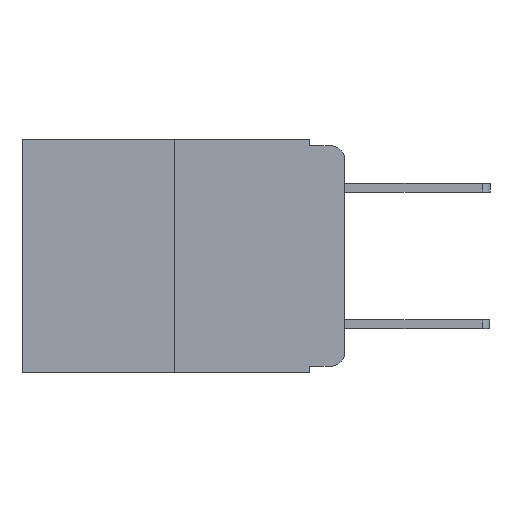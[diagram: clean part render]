
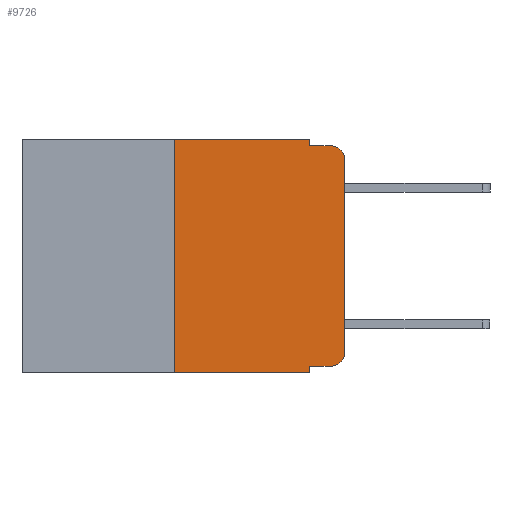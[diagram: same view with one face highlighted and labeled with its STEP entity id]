
A CAD part, left-side view. The second image highlights one B-rep face of the part: STEP entity #9726.
In plain terms, the highlighted planar face has unit normal (-1, 0, 0).
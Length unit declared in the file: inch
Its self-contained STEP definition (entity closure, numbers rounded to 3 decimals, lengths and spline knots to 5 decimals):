
#6 = EDGE_LOOP ( 'NONE', ( #5676, #11963, #8001, #12104, #3830, #6440, #8475, #7396, #10908, #8155 ) ) ;
#300 = FACE_OUTER_BOUND ( 'NONE', #6, .T. ) ;
#561 = VERTEX_POINT ( 'NONE', #10012 ) ;
#923 = CARTESIAN_POINT ( 'NONE',  ( 0., 0.473, -0.343 ) ) ;
#1143 = AXIS2_PLACEMENT_3D ( 'NONE', #9100, #2590, #10168 ) ;
#1240 = CARTESIAN_POINT ( 'NONE',  ( 0., 0.02, -0.03 ) ) ;
#1515 = DIRECTION ( 'NONE',  ( 0., -1., 0. ) ) ;
#1975 = LINE ( 'NONE', #8167, #10622 ) ;
#2472 = DIRECTION ( 'NONE',  ( 0., 0., -1. ) ) ;
#2590 = DIRECTION ( 'NONE',  ( -1., 0., 0. ) ) ;
#2690 = CARTESIAN_POINT ( 'NONE',  ( 0., 0.051, -0.333 ) ) ;
#2738 = VECTOR ( 'NONE', #5827, 39.37008 ) ;
#3162 = VERTEX_POINT ( 'NONE', #2690 ) ;
#3560 = CARTESIAN_POINT ( 'NONE',  ( 0., 0.02, -0.333 ) ) ;
#3591 = VERTEX_POINT ( 'NONE', #3560 ) ;
#3830 = ORIENTED_EDGE ( 'NONE', *, *, #11233, .F. ) ;
#3986 = PLANE ( 'NONE',  #9888 ) ;
#4048 = CIRCLE ( 'NONE', #1143, 0.02 ) ;
#4420 = LINE ( 'NONE', #9017, #10023 ) ;
#4457 = LINE ( 'NONE', #7107, #9730 ) ;
#4515 = DIRECTION ( 'NONE',  ( 0., -1., 0. ) ) ;
#4577 = EDGE_CURVE ( 'NONE', #561, #8342, #7917, .T. ) ;
#4603 = EDGE_CURVE ( 'NONE', #12995, #8988, #4457, .T. ) ;
#4677 = CARTESIAN_POINT ( 'NONE',  ( 0., 0.051, 0. ) ) ;
#4731 = CARTESIAN_POINT ( 'NONE',  ( 0., 0.051, 0. ) ) ;
#4931 = CARTESIAN_POINT ( 'NONE',  ( 0., 0.25, 0. ) ) ;
#5066 = VERTEX_POINT ( 'NONE', #13216 ) ;
#5166 = DIRECTION ( 'NONE',  ( 1., 0., 0. ) ) ;
#5262 = EDGE_CURVE ( 'NONE', #9097, #7649, #11255, .T. ) ;
#5288 = EDGE_CURVE ( 'NONE', #3162, #8228, #13524, .T. ) ;
#5335 = EDGE_CURVE ( 'NONE', #3162, #3591, #4420, .T. ) ;
#5362 = EDGE_CURVE ( 'NONE', #3591, #12995, #4048, .T. ) ;
#5676 = ORIENTED_EDGE ( 'NONE', *, *, #4603, .T. ) ;
#5827 = DIRECTION ( 'NONE',  ( 0., 0., -1. ) ) ;
#5841 = CARTESIAN_POINT ( 'NONE',  ( 0., 0.051, -0.01 ) ) ;
#6189 = CARTESIAN_POINT ( 'NONE',  ( 0., 0.473, 0. ) ) ;
#6440 = ORIENTED_EDGE ( 'NONE', *, *, #4577, .F. ) ;
#6747 = CIRCLE ( 'NONE', #13376, 0.02 ) ;
#7107 = CARTESIAN_POINT ( 'NONE',  ( 0., 0., 0. ) ) ;
#7198 = CARTESIAN_POINT ( 'NONE',  ( 0., 0.051, -0.343 ) ) ;
#7371 = CARTESIAN_POINT ( 'NONE',  ( 0., 0.25, 0. ) ) ;
#7396 = ORIENTED_EDGE ( 'NONE', *, *, #5288, .F. ) ;
#7463 = CARTESIAN_POINT ( 'NONE',  ( 0., 0., -0.313 ) ) ;
#7619 = VECTOR ( 'NONE', #10121, 39.37008 ) ;
#7649 = VERTEX_POINT ( 'NONE', #5841 ) ;
#7884 = VECTOR ( 'NONE', #11900, 39.37008 ) ;
#7917 = LINE ( 'NONE', #4931, #7619 ) ;
#8001 = ORIENTED_EDGE ( 'NONE', *, *, #11429, .F. ) ;
#8015 = VECTOR ( 'NONE', #12577, 39.37008 ) ;
#8155 = ORIENTED_EDGE ( 'NONE', *, *, #5362, .T. ) ;
#8167 = CARTESIAN_POINT ( 'NONE',  ( 0., 0.473, 0. ) ) ;
#8228 = VERTEX_POINT ( 'NONE', #7198 ) ;
#8342 = VERTEX_POINT ( 'NONE', #7371 ) ;
#8475 = ORIENTED_EDGE ( 'NONE', *, *, #8491, .T. ) ;
#8491 = EDGE_CURVE ( 'NONE', #561, #8228, #11672, .T. ) ;
#8737 = DIRECTION ( 'NONE',  ( 0., -1., 0. ) ) ;
#8988 = VERTEX_POINT ( 'NONE', #12759 ) ;
#9004 = DIRECTION ( 'NONE',  ( -1., 0., 0. ) ) ;
#9017 = CARTESIAN_POINT ( 'NONE',  ( 0., 0.051, -0.333 ) ) ;
#9097 = VERTEX_POINT ( 'NONE', #13017 ) ;
#9100 = CARTESIAN_POINT ( 'NONE',  ( 0., 0.02, -0.313 ) ) ;
#9316 = VECTOR ( 'NONE', #8737, 39.37008 ) ;
#9726 = ADVANCED_FACE ( 'NONE', ( #300 ), #3986, .F. ) ;
#9730 = VECTOR ( 'NONE', #13111, 39.37008 ) ;
#9888 = AXIS2_PLACEMENT_3D ( 'NONE', #6189, #5166, #12253 ) ;
#10012 = CARTESIAN_POINT ( 'NONE',  ( 0., 0.25, -0.343 ) ) ;
#10023 = VECTOR ( 'NONE', #4515, 39.37008 ) ;
#10121 = DIRECTION ( 'NONE',  ( 0., 0., 1. ) ) ;
#10168 = DIRECTION ( 'NONE',  ( 0., 0., -1. ) ) ;
#10622 = VECTOR ( 'NONE', #1515, 39.37008 ) ;
#10908 = ORIENTED_EDGE ( 'NONE', *, *, #5335, .T. ) ;
#11233 = EDGE_CURVE ( 'NONE', #8342, #9097, #1975, .T. ) ;
#11255 = LINE ( 'NONE', #4677, #2738 ) ;
#11429 = EDGE_CURVE ( 'NONE', #7649, #5066, #13071, .T. ) ;
#11653 = CARTESIAN_POINT ( 'NONE',  ( 0., 0.051, -0.01 ) ) ;
#11672 = LINE ( 'NONE', #923, #9316 ) ;
#11900 = DIRECTION ( 'NONE',  ( 0., 0., -1. ) ) ;
#11963 = ORIENTED_EDGE ( 'NONE', *, *, #12152, .T. ) ;
#12104 = ORIENTED_EDGE ( 'NONE', *, *, #5262, .F. ) ;
#12152 = EDGE_CURVE ( 'NONE', #8988, #5066, #6747, .T. ) ;
#12253 = DIRECTION ( 'NONE',  ( 0., 0., -1. ) ) ;
#12577 = DIRECTION ( 'NONE',  ( 0., -1., 0. ) ) ;
#12759 = CARTESIAN_POINT ( 'NONE',  ( 0., 0., -0.03 ) ) ;
#12995 = VERTEX_POINT ( 'NONE', #7463 ) ;
#13017 = CARTESIAN_POINT ( 'NONE',  ( 0., 0.051, 0. ) ) ;
#13071 = LINE ( 'NONE', #11653, #8015 ) ;
#13111 = DIRECTION ( 'NONE',  ( 0., 0., 1. ) ) ;
#13216 = CARTESIAN_POINT ( 'NONE',  ( 0., 0.02, -0.01 ) ) ;
#13376 = AXIS2_PLACEMENT_3D ( 'NONE', #1240, #9004, #2472 ) ;
#13524 = LINE ( 'NONE', #4731, #7884 ) ;
